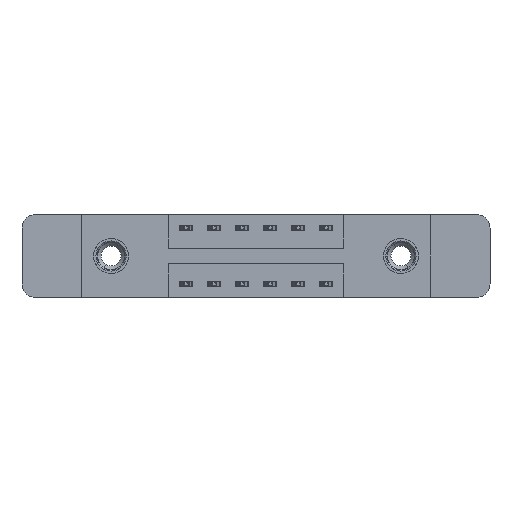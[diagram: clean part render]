
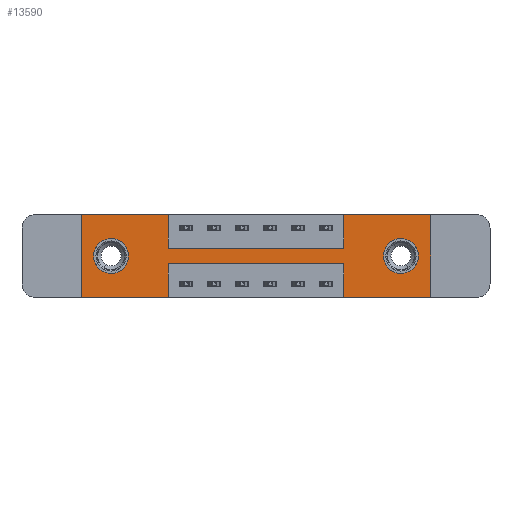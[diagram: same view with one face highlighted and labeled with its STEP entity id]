
A CAD part, front view. The second image highlights one B-rep face of the part: STEP entity #13590.
In plain terms, the highlighted planar face has unit normal (0, -1, 0).
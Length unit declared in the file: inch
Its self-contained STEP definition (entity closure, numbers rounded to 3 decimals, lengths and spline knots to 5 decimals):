
#284 = VERTEX_POINT ( 'NONE', #5384 ) ;
#376 = CARTESIAN_POINT ( 'NONE',  ( 0.3875, 0., -0.15 ) ) ;
#451 = CARTESIAN_POINT ( 'NONE',  ( 1.4275, 0., -0.185 ) ) ;
#927 = VECTOR ( 'NONE', #12898, 39.37008 ) ;
#972 = DIRECTION ( 'NONE',  ( 0., 0., -1. ) ) ;
#974 = CARTESIAN_POINT ( 'NONE',  ( 0., 0., -0.37 ) ) ;
#1020 = EDGE_CURVE ( 'NONE', #10211, #5041, #5291, .T. ) ;
#1113 = EDGE_CURVE ( 'NONE', #284, #1302, #7491, .T. ) ;
#1212 = EDGE_LOOP ( 'NONE', ( #13920, #11469 ) ) ;
#1302 = VERTEX_POINT ( 'NONE', #376 ) ;
#1335 = DIRECTION ( 'NONE',  ( 0., 1., 0. ) ) ;
#1352 = EDGE_CURVE ( 'NONE', #3742, #6206, #2625, .T. ) ;
#1456 = DIRECTION ( 'NONE',  ( 0., 0., -1. ) ) ;
#1507 = EDGE_CURVE ( 'NONE', #1302, #3421, #6821, .T. ) ;
#1646 = EDGE_LOOP ( 'NONE', ( #7501, #13852 ) ) ;
#1716 = CARTESIAN_POINT ( 'NONE',  ( 0., 0., 0. ) ) ;
#1743 = EDGE_CURVE ( 'NONE', #2409, #7583, #12395, .T. ) ;
#1873 = ORIENTED_EDGE ( 'NONE', *, *, #1113, .F. ) ;
#1991 = ORIENTED_EDGE ( 'NONE', *, *, #12765, .F. ) ;
#2187 = VECTOR ( 'NONE', #3181, 39.37008 ) ;
#2299 = DIRECTION ( 'NONE',  ( 0., 0., -1. ) ) ;
#2409 = VERTEX_POINT ( 'NONE', #10117 ) ;
#2625 = LINE ( 'NONE', #5711, #7653 ) ;
#2776 = CARTESIAN_POINT ( 'NONE',  ( 0.3875, 0., -0.37 ) ) ;
#3168 = ORIENTED_EDGE ( 'NONE', *, *, #1352, .F. ) ;
#3181 = DIRECTION ( 'NONE',  ( -1., 0., 0. ) ) ;
#3218 = DIRECTION ( 'NONE',  ( 0., 1., 0. ) ) ;
#3238 = VERTEX_POINT ( 'NONE', #9821 ) ;
#3281 = CARTESIAN_POINT ( 'NONE',  ( 1.1725, 0., -0.15 ) ) ;
#3386 = CARTESIAN_POINT ( 'NONE',  ( 0.3875, 0., 0. ) ) ;
#3421 = VERTEX_POINT ( 'NONE', #3281 ) ;
#3498 = CARTESIAN_POINT ( 'NONE',  ( 0.1325, 0., -0.185 ) ) ;
#3684 = VERTEX_POINT ( 'NONE', #9632 ) ;
#3742 = VERTEX_POINT ( 'NONE', #9727 ) ;
#4002 = FACE_BOUND ( 'NONE', #1646, .T. ) ;
#4177 = DIRECTION ( 'NONE',  ( 0., 0., 1. ) ) ;
#4478 = CARTESIAN_POINT ( 'NONE',  ( 0., 0., 0. ) ) ;
#4595 = CIRCLE ( 'NONE', #7632, 0.078 ) ;
#4623 = DIRECTION ( 'NONE',  ( 0., 1., 0. ) ) ;
#4901 = DIRECTION ( 'NONE',  ( 0., 1., 0. ) ) ;
#4949 = ORIENTED_EDGE ( 'NONE', *, *, #6044, .F. ) ;
#5021 = FACE_OUTER_BOUND ( 'NONE', #8760, .T. ) ;
#5041 = VERTEX_POINT ( 'NONE', #4478 ) ;
#5161 = CIRCLE ( 'NONE', #13512, 0.078 ) ;
#5188 = VECTOR ( 'NONE', #10689, 39.37008 ) ;
#5218 = CARTESIAN_POINT ( 'NONE',  ( 1.4275, 0., -0.185 ) ) ;
#5233 = CARTESIAN_POINT ( 'NONE',  ( 1.4275, 0., -0.107 ) ) ;
#5291 = LINE ( 'NONE', #6230, #13254 ) ;
#5363 = LINE ( 'NONE', #8833, #10954 ) ;
#5384 = CARTESIAN_POINT ( 'NONE',  ( 0.3875, 0., 0. ) ) ;
#5466 = CARTESIAN_POINT ( 'NONE',  ( 0., 0., -0.37 ) ) ;
#5634 = AXIS2_PLACEMENT_3D ( 'NONE', #451, #4623, #9990 ) ;
#5671 = CARTESIAN_POINT ( 'NONE',  ( 1.1725, 0., 0. ) ) ;
#5709 = LINE ( 'NONE', #2776, #6021 ) ;
#5711 = CARTESIAN_POINT ( 'NONE',  ( 1.56, 0., 0. ) ) ;
#5880 = CARTESIAN_POINT ( 'NONE',  ( 0.1325, 0., -0.185 ) ) ;
#6021 = VECTOR ( 'NONE', #11386, 39.37008 ) ;
#6024 = DIRECTION ( 'NONE',  ( 0., 0., 1. ) ) ;
#6044 = EDGE_CURVE ( 'NONE', #9033, #10211, #7058, .T. ) ;
#6116 = AXIS2_PLACEMENT_3D ( 'NONE', #7839, #12202, #8919 ) ;
#6206 = VERTEX_POINT ( 'NONE', #6631 ) ;
#6230 = CARTESIAN_POINT ( 'NONE',  ( 0., 0., 0. ) ) ;
#6470 = EDGE_CURVE ( 'NONE', #5041, #284, #7550, .T. ) ;
#6596 = VERTEX_POINT ( 'NONE', #11213 ) ;
#6631 = CARTESIAN_POINT ( 'NONE',  ( 1.56, 0., -0.37 ) ) ;
#6740 = DIRECTION ( 'NONE',  ( -1., 0., 0. ) ) ;
#6778 = EDGE_CURVE ( 'NONE', #10551, #3742, #10066, .T. ) ;
#6821 = LINE ( 'NONE', #9754, #927 ) ;
#6893 = LINE ( 'NONE', #8111, #13329 ) ;
#6975 = EDGE_CURVE ( 'NONE', #11183, #8465, #5161, .T. ) ;
#7058 = LINE ( 'NONE', #974, #5188 ) ;
#7143 = LINE ( 'NONE', #8240, #9173 ) ;
#7346 = CARTESIAN_POINT ( 'NONE',  ( 0.1325, 0., -0.107 ) ) ;
#7410 = ORIENTED_EDGE ( 'NONE', *, *, #1507, .F. ) ;
#7491 = LINE ( 'NONE', #3386, #9692 ) ;
#7501 = ORIENTED_EDGE ( 'NONE', *, *, #13707, .T. ) ;
#7550 = LINE ( 'NONE', #1716, #11437 ) ;
#7552 = CARTESIAN_POINT ( 'NONE',  ( 0., 0., 0. ) ) ;
#7583 = VERTEX_POINT ( 'NONE', #5233 ) ;
#7632 = AXIS2_PLACEMENT_3D ( 'NONE', #3498, #1335, #4177 ) ;
#7653 = VECTOR ( 'NONE', #1456, 39.37008 ) ;
#7839 = CARTESIAN_POINT ( 'NONE',  ( 0., 0., -0.37 ) ) ;
#7963 = ORIENTED_EDGE ( 'NONE', *, *, #11828, .F. ) ;
#8018 = ORIENTED_EDGE ( 'NONE', *, *, #6470, .F. ) ;
#8019 = DIRECTION ( 'NONE',  ( 0., 0., 1. ) ) ;
#8084 = ORIENTED_EDGE ( 'NONE', *, *, #12583, .F. ) ;
#8111 = CARTESIAN_POINT ( 'NONE',  ( 1.1725, 0., -0.37 ) ) ;
#8230 = LINE ( 'NONE', #5466, #2187 ) ;
#8240 = CARTESIAN_POINT ( 'NONE',  ( 1.1725, 0., 0. ) ) ;
#8374 = EDGE_CURVE ( 'NONE', #3421, #10551, #7143, .T. ) ;
#8465 = VERTEX_POINT ( 'NONE', #7346 ) ;
#8487 = CARTESIAN_POINT ( 'NONE',  ( 0.3875, 0., -0.37 ) ) ;
#8514 = DIRECTION ( 'NONE',  ( 1., 0., 0. ) ) ;
#8760 = EDGE_LOOP ( 'NONE', ( #8084, #7963, #1991, #11423, #3168, #9181, #10493, #7410, #1873, #8018, #13349, #4949 ) ) ;
#8833 = CARTESIAN_POINT ( 'NONE',  ( 0.3875, 0., -0.22 ) ) ;
#8873 = PLANE ( 'NONE',  #6116 ) ;
#8919 = DIRECTION ( 'NONE',  ( 0., 0., -1. ) ) ;
#9033 = VERTEX_POINT ( 'NONE', #8487 ) ;
#9054 = VECTOR ( 'NONE', #8514, 39.37008 ) ;
#9173 = VECTOR ( 'NONE', #6024, 39.37008 ) ;
#9181 = ORIENTED_EDGE ( 'NONE', *, *, #6778, .F. ) ;
#9552 = AXIS2_PLACEMENT_3D ( 'NONE', #5218, #3218, #972 ) ;
#9632 = CARTESIAN_POINT ( 'NONE',  ( 1.1725, 0., -0.37 ) ) ;
#9661 = EDGE_CURVE ( 'NONE', #8465, #11183, #4595, .T. ) ;
#9692 = VECTOR ( 'NONE', #2299, 39.37008 ) ;
#9727 = CARTESIAN_POINT ( 'NONE',  ( 1.56, 0., 0. ) ) ;
#9754 = CARTESIAN_POINT ( 'NONE',  ( 0.3875, 0., -0.15 ) ) ;
#9821 = CARTESIAN_POINT ( 'NONE',  ( 1.1725, 0., -0.22 ) ) ;
#9843 = CARTESIAN_POINT ( 'NONE',  ( 0., 0., -0.37 ) ) ;
#9990 = DIRECTION ( 'NONE',  ( 0., 0., -1. ) ) ;
#10066 = LINE ( 'NONE', #7552, #9054 ) ;
#10117 = CARTESIAN_POINT ( 'NONE',  ( 1.4275, 0., -0.263 ) ) ;
#10211 = VERTEX_POINT ( 'NONE', #9843 ) ;
#10242 = DIRECTION ( 'NONE',  ( 1., 0., 0. ) ) ;
#10493 = ORIENTED_EDGE ( 'NONE', *, *, #8374, .F. ) ;
#10551 = VERTEX_POINT ( 'NONE', #5671 ) ;
#10689 = DIRECTION ( 'NONE',  ( -1., 0., 0. ) ) ;
#10765 = DIRECTION ( 'NONE',  ( 0., 0., 1. ) ) ;
#10954 = VECTOR ( 'NONE', #6740, 39.37008 ) ;
#11183 = VERTEX_POINT ( 'NONE', #13173 ) ;
#11213 = CARTESIAN_POINT ( 'NONE',  ( 0.3875, 0., -0.22 ) ) ;
#11357 = DIRECTION ( 'NONE',  ( 0., 0., 1. ) ) ;
#11386 = DIRECTION ( 'NONE',  ( 0., 0., -1. ) ) ;
#11423 = ORIENTED_EDGE ( 'NONE', *, *, #12684, .F. ) ;
#11437 = VECTOR ( 'NONE', #10242, 39.37008 ) ;
#11469 = ORIENTED_EDGE ( 'NONE', *, *, #6975, .T. ) ;
#11828 = EDGE_CURVE ( 'NONE', #3238, #6596, #5363, .T. ) ;
#12202 = DIRECTION ( 'NONE',  ( 0., -1., 0. ) ) ;
#12298 = FACE_BOUND ( 'NONE', #1212, .T. ) ;
#12395 = CIRCLE ( 'NONE', #5634, 0.078 ) ;
#12583 = EDGE_CURVE ( 'NONE', #6596, #9033, #5709, .T. ) ;
#12684 = EDGE_CURVE ( 'NONE', #6206, #3684, #8230, .T. ) ;
#12765 = EDGE_CURVE ( 'NONE', #3684, #3238, #6893, .T. ) ;
#12898 = DIRECTION ( 'NONE',  ( 1., 0., 0. ) ) ;
#13173 = CARTESIAN_POINT ( 'NONE',  ( 0.1325, 0., -0.263 ) ) ;
#13254 = VECTOR ( 'NONE', #10765, 39.37008 ) ;
#13329 = VECTOR ( 'NONE', #8019, 39.37008 ) ;
#13349 = ORIENTED_EDGE ( 'NONE', *, *, #1020, .F. ) ;
#13512 = AXIS2_PLACEMENT_3D ( 'NONE', #5880, #4901, #11357 ) ;
#13590 = ADVANCED_FACE ( 'NONE', ( #4002, #12298, #5021 ), #8873, .T. ) ;
#13638 = CIRCLE ( 'NONE', #9552, 0.078 ) ;
#13707 = EDGE_CURVE ( 'NONE', #7583, #2409, #13638, .T. ) ;
#13852 = ORIENTED_EDGE ( 'NONE', *, *, #1743, .T. ) ;
#13920 = ORIENTED_EDGE ( 'NONE', *, *, #9661, .T. ) ;
